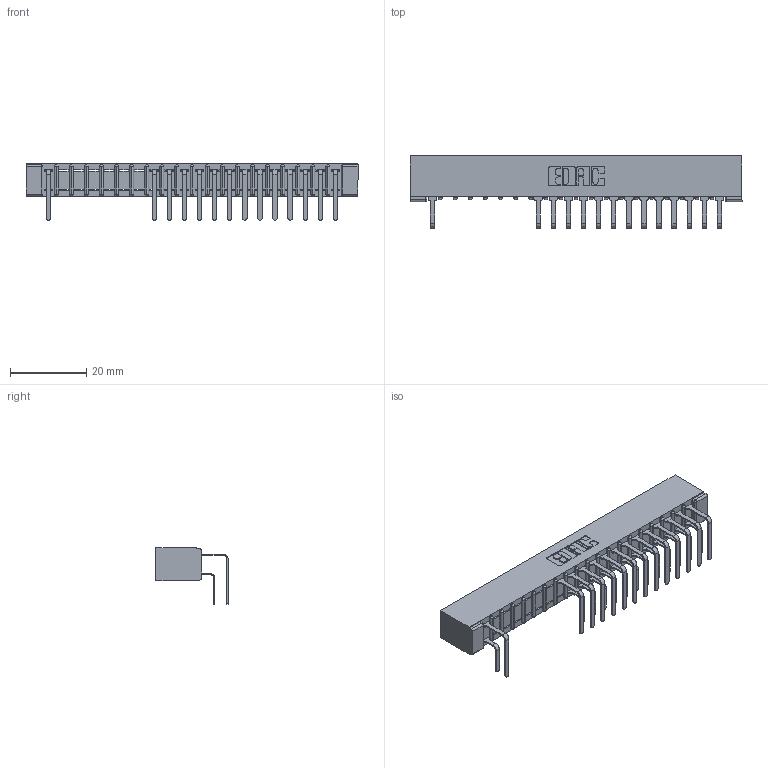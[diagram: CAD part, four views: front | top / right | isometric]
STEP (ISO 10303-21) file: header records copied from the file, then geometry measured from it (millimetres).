
FILE_DESCRIPTION (( 'STEP AP203' ), '1' );
FILE_NAME ('307-040-558-201.STEP', '2018-08-05T15:09:05', ( '' ), ( '' ), 'SwSTEP 2.0', 'SolidWorks 2016', '' );
FILE_SCHEMA (( 'CONFIG_CONTROL_DESIGN' ));
Length unit declared in the file: inch
Products named in the file (4): 307 Part_No Mounting Lugs; 307-290-001_558 559 - 1 (Single); 307-290-001_558 - 2 (Single); 307-040-558-201
Assembly tree (28 placements, depth 2):
  307-040-558-201
    307 Part_No Mounting Lugs
    307-290-001_558 559 - 1 (Single)  x13
    307-290-001_558 - 2 (Single)  x14
Bounding box: 87.12 x 18.96 x 14.81 mm (x, y, z)
Volume: 5885.1 mm3; surface area: 10450.7 mm2
Topology: 28 solids, 28 shells, 1611 faces, 4549 edges, 2938 vertices
Faces by surface type: plane 1035, cylinder 534, sphere 42
Entity records: 21251 total; most frequent: CARTESIAN_POINT 3537, ORIENTED_EDGE 3514, DIRECTION 3459, EDGE_CURVE 1757, VECTOR 1339, LINE 1339, VERTEX_POINT 1138, AXIS2_PLACEMENT_3D 1060
